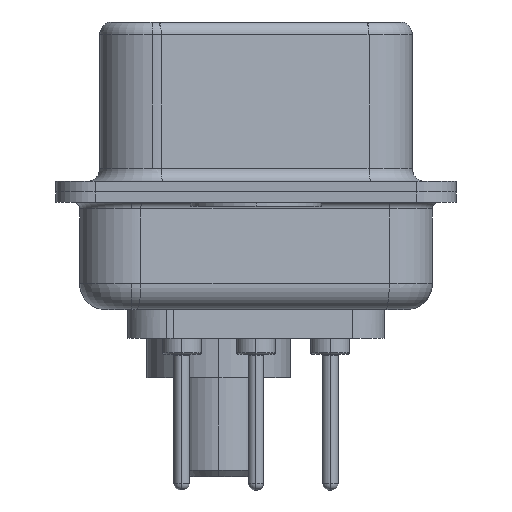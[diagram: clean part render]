
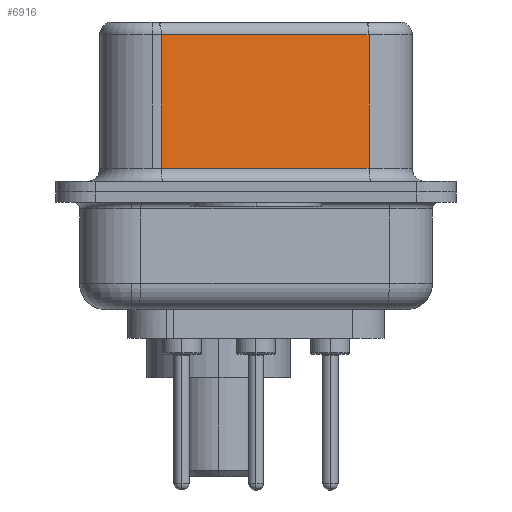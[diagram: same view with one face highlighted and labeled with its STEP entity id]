
A CAD part, left-side view. The second image highlights one B-rep face of the part: STEP entity #6916.
In plain terms, the highlighted planar face has unit normal (-0.985, -0.174, 0).
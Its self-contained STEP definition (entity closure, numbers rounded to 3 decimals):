
#50 = LINE ( 'NONE', #21223, #10220 ) ;
#708 = DIRECTION ( 'NONE',  ( -0.174, 0.985, 0. ) ) ;
#3079 = VECTOR ( 'NONE', #15370, 1000. ) ;
#3160 = EDGE_CURVE ( 'NONE', #7279, #19354, #19246, .T. ) ;
#3679 = ORIENTED_EDGE ( 'NONE', *, *, #23343, .T. ) ;
#4895 = CARTESIAN_POINT ( 'NONE',  ( 5.132, -4.322, 6.02 ) ) ;
#5329 = CARTESIAN_POINT ( 'NONE',  ( 5.132, -4.322, 0.9 ) ) ;
#6916 = ADVANCED_FACE ( 'NONE', ( #22748 ), #17730, .F. ) ;
#7122 = ORIENTED_EDGE ( 'NONE', *, *, #3160, .T. ) ;
#7279 = VERTEX_POINT ( 'NONE', #4895 ) ;
#7658 = EDGE_LOOP ( 'NONE', ( #12294, #7122, #3679, #7971 ) ) ;
#7971 = ORIENTED_EDGE ( 'NONE', *, *, #14621, .T. ) ;
#9522 = VERTEX_POINT ( 'NONE', #18804 ) ;
#10220 = VECTOR ( 'NONE', #23313, 1000. ) ;
#10322 = AXIS2_PLACEMENT_3D ( 'NONE', #18023, #17452, #17418 ) ;
#10341 = VERTEX_POINT ( 'NONE', #15226 ) ;
#11416 = VECTOR ( 'NONE', #19381, 1000. ) ;
#12294 = ORIENTED_EDGE ( 'NONE', *, *, #21486, .F. ) ;
#13319 = CARTESIAN_POINT ( 'NONE',  ( 3.73, 3.628, 6.02 ) ) ;
#13745 = LINE ( 'NONE', #23490, #3079 ) ;
#14621 = EDGE_CURVE ( 'NONE', #10341, #9522, #17401, .T. ) ;
#15226 = CARTESIAN_POINT ( 'NONE',  ( 3.73, 3.628, 0.9 ) ) ;
#15370 = DIRECTION ( 'NONE',  ( 0., 0., -1. ) ) ;
#17401 = LINE ( 'NONE', #5329, #11416 ) ;
#17418 = DIRECTION ( 'NONE',  ( -0.174, 0.985, 0. ) ) ;
#17452 = DIRECTION ( 'NONE',  ( 0.985, 0.174, 0. ) ) ;
#17730 = PLANE ( 'NONE',  #10322 ) ;
#18023 = CARTESIAN_POINT ( 'NONE',  ( 5.132, -4.322, 6.52 ) ) ;
#18804 = CARTESIAN_POINT ( 'NONE',  ( 5.132, -4.322, 0.9 ) ) ;
#19246 = LINE ( 'NONE', #22090, #19887 ) ;
#19354 = VERTEX_POINT ( 'NONE', #13319 ) ;
#19381 = DIRECTION ( 'NONE',  ( 0.174, -0.985, 0. ) ) ;
#19887 = VECTOR ( 'NONE', #708, 1000. ) ;
#21223 = CARTESIAN_POINT ( 'NONE',  ( 3.73, 3.628, 6.52 ) ) ;
#21486 = EDGE_CURVE ( 'NONE', #7279, #9522, #13745, .T. ) ;
#22090 = CARTESIAN_POINT ( 'NONE',  ( 5.132, -4.322, 6.02 ) ) ;
#22748 = FACE_OUTER_BOUND ( 'NONE', #7658, .T. ) ;
#23313 = DIRECTION ( 'NONE',  ( 0., 0., -1. ) ) ;
#23343 = EDGE_CURVE ( 'NONE', #19354, #10341, #50, .T. ) ;
#23490 = CARTESIAN_POINT ( 'NONE',  ( 5.132, -4.322, 6.52 ) ) ;
